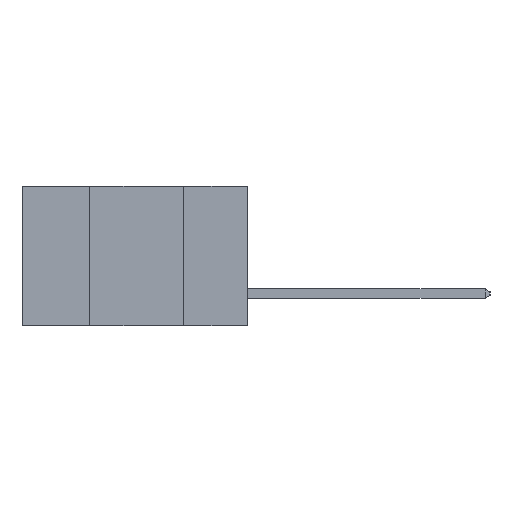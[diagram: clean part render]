
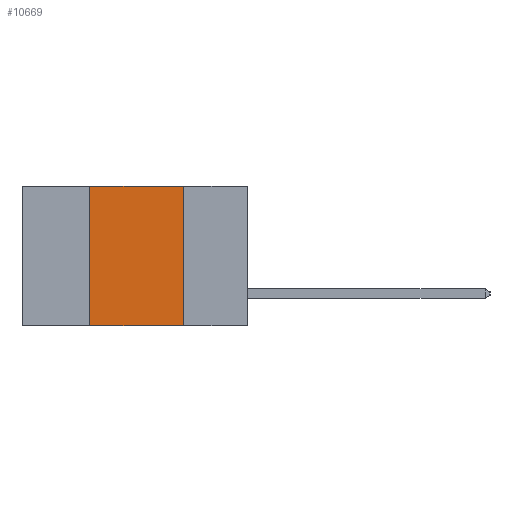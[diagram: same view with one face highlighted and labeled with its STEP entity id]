
A CAD part, left-side view. The second image highlights one B-rep face of the part: STEP entity #10669.
In plain terms, the highlighted planar face has unit normal (-1, 0, 0).
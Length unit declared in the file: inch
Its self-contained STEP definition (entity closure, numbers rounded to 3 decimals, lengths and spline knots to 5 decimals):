
#543 = CARTESIAN_POINT ( 'NONE',  ( 0., 0.17, 0. ) ) ;
#652 = VERTEX_POINT ( 'NONE', #2709 ) ;
#753 = DIRECTION ( 'NONE',  ( 0., -1., 0. ) ) ;
#1034 = EDGE_LOOP ( 'NONE', ( #5354, #8334, #8309, #6332 ) ) ;
#1457 = VERTEX_POINT ( 'NONE', #543 ) ;
#1843 = CARTESIAN_POINT ( 'NONE',  ( 0., 0.6, 0. ) ) ;
#2270 = EDGE_CURVE ( 'NONE', #652, #6399, #3853, .T. ) ;
#2616 = EDGE_CURVE ( 'NONE', #652, #10859, #13722, .T. ) ;
#2709 = CARTESIAN_POINT ( 'NONE',  ( 0., 0.42, -0.37 ) ) ;
#2801 = EDGE_CURVE ( 'NONE', #1457, #6399, #11170, .T. ) ;
#3090 = VECTOR ( 'NONE', #7152, 39.37008 ) ;
#3853 = LINE ( 'NONE', #12668, #3090 ) ;
#4240 = VECTOR ( 'NONE', #4461, 39.37008 ) ;
#4284 = DIRECTION ( 'NONE',  ( 0., 0., -1. ) ) ;
#4461 = DIRECTION ( 'NONE',  ( 0., 0., 1. ) ) ;
#5022 = CARTESIAN_POINT ( 'NONE',  ( 0., 0.42, 0. ) ) ;
#5354 = ORIENTED_EDGE ( 'NONE', *, *, #2801, .F. ) ;
#5510 = CARTESIAN_POINT ( 'NONE',  ( 0., 0.17, 0. ) ) ;
#6332 = ORIENTED_EDGE ( 'NONE', *, *, #2270, .T. ) ;
#6399 = VERTEX_POINT ( 'NONE', #12073 ) ;
#7152 = DIRECTION ( 'NONE',  ( 0., -1., 0. ) ) ;
#7997 = VECTOR ( 'NONE', #14647, 39.37008 ) ;
#8309 = ORIENTED_EDGE ( 'NONE', *, *, #2616, .F. ) ;
#8334 = ORIENTED_EDGE ( 'NONE', *, *, #10724, .F. ) ;
#9063 = PLANE ( 'NONE',  #10934 ) ;
#10669 = ADVANCED_FACE ( 'NONE', ( #15105 ), #9063, .F. ) ;
#10724 = EDGE_CURVE ( 'NONE', #10859, #1457, #14033, .T. ) ;
#10859 = VERTEX_POINT ( 'NONE', #12926 ) ;
#10934 = AXIS2_PLACEMENT_3D ( 'NONE', #1843, #11465, #4284 ) ;
#10970 = VECTOR ( 'NONE', #753, 39.37008 ) ;
#11170 = LINE ( 'NONE', #5510, #7997 ) ;
#11465 = DIRECTION ( 'NONE',  ( 1., 0., 0. ) ) ;
#11512 = CARTESIAN_POINT ( 'NONE',  ( 0., 0.6, 0. ) ) ;
#12073 = CARTESIAN_POINT ( 'NONE',  ( 0., 0.17, -0.37 ) ) ;
#12668 = CARTESIAN_POINT ( 'NONE',  ( 0., 0.6, -0.37 ) ) ;
#12926 = CARTESIAN_POINT ( 'NONE',  ( 0., 0.42, 0. ) ) ;
#13722 = LINE ( 'NONE', #5022, #4240 ) ;
#14033 = LINE ( 'NONE', #11512, #10970 ) ;
#14647 = DIRECTION ( 'NONE',  ( 0., 0., -1. ) ) ;
#15105 = FACE_OUTER_BOUND ( 'NONE', #1034, .T. ) ;
